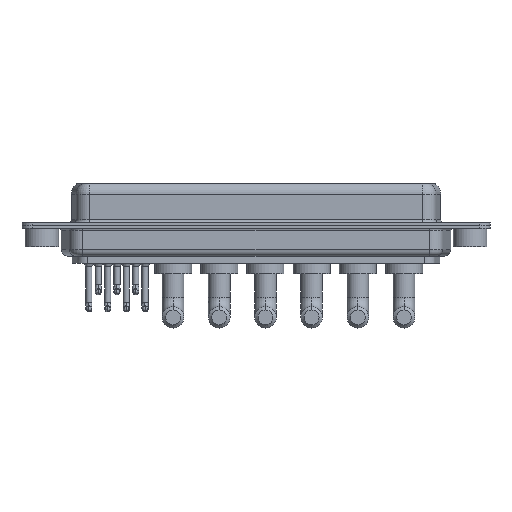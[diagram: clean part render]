
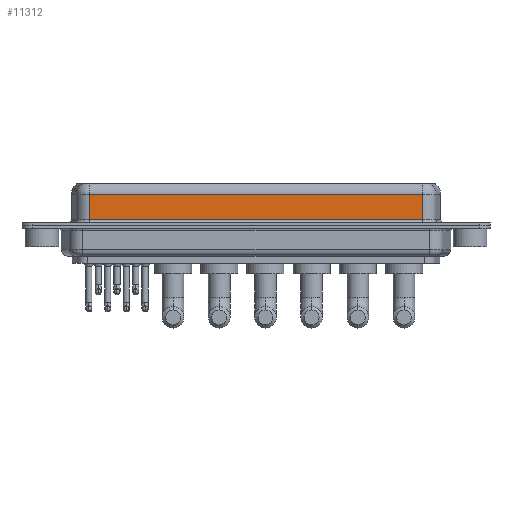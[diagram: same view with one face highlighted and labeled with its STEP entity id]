
A CAD part, front view. The second image highlights one B-rep face of the part: STEP entity #11312.
In plain terms, the highlighted planar face has unit normal (0, -1, 0).
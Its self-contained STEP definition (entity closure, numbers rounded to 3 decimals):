
#74 = LINE ( 'NONE', #2670, #17532 ) ;
#169 = VERTEX_POINT ( 'NONE', #14620 ) ;
#1276 = DIRECTION ( 'NONE',  ( 0., 0., -1. ) ) ;
#1426 = DIRECTION ( 'NONE',  ( -1., 0., 0. ) ) ;
#1740 = EDGE_CURVE ( 'NONE', #11932, #169, #18447, .T. ) ;
#2670 = CARTESIAN_POINT ( 'NONE',  ( 56.462, -3.95, 6.4 ) ) ;
#2834 = CARTESIAN_POINT ( 'NONE',  ( 56.462, -3.95, 4.65 ) ) ;
#3176 = VERTEX_POINT ( 'NONE', #13389 ) ;
#3404 = DIRECTION ( 'NONE',  ( 1., 0., 0. ) ) ;
#3586 = CARTESIAN_POINT ( 'NONE',  ( 56.462, -3.95, 0.9 ) ) ;
#4242 = VERTEX_POINT ( 'NONE', #7352 ) ;
#5449 = AXIS2_PLACEMENT_3D ( 'NONE', #15135, #15228, #6445 ) ;
#5517 = EDGE_CURVE ( 'NONE', #11932, #4242, #74, .T. ) ;
#5564 = EDGE_LOOP ( 'NONE', ( #15356, #7117, #18203, #12481 ) ) ;
#6445 = DIRECTION ( 'NONE',  ( 0., 0., 1. ) ) ;
#6584 = VECTOR ( 'NONE', #13882, 1000. ) ;
#7117 = ORIENTED_EDGE ( 'NONE', *, *, #1740, .T. ) ;
#7352 = CARTESIAN_POINT ( 'NONE',  ( 56.462, -3.95, 0.9 ) ) ;
#7949 = PLANE ( 'NONE',  #5449 ) ;
#8182 = EDGE_CURVE ( 'NONE', #169, #3176, #11280, .T. ) ;
#8204 = VECTOR ( 'NONE', #1426, 1000. ) ;
#8473 = EDGE_CURVE ( 'NONE', #3176, #4242, #16222, .T. ) ;
#9725 = FACE_OUTER_BOUND ( 'NONE', #5564, .T. ) ;
#11210 = CARTESIAN_POINT ( 'NONE',  ( 56.462, -3.95, 4.65 ) ) ;
#11280 = LINE ( 'NONE', #16697, #6584 ) ;
#11312 = ADVANCED_FACE ( 'NONE', ( #9725 ), #7949, .F. ) ;
#11932 = VERTEX_POINT ( 'NONE', #11210 ) ;
#12481 = ORIENTED_EDGE ( 'NONE', *, *, #8473, .T. ) ;
#13389 = CARTESIAN_POINT ( 'NONE',  ( 7.038, -3.95, 0.9 ) ) ;
#13882 = DIRECTION ( 'NONE',  ( 0., 0., -1. ) ) ;
#14327 = VECTOR ( 'NONE', #3404, 1000. ) ;
#14620 = CARTESIAN_POINT ( 'NONE',  ( 7.038, -3.95, 4.65 ) ) ;
#15135 = CARTESIAN_POINT ( 'NONE',  ( 56.462, -3.95, 6.4 ) ) ;
#15228 = DIRECTION ( 'NONE',  ( 0., 1., 0. ) ) ;
#15356 = ORIENTED_EDGE ( 'NONE', *, *, #5517, .F. ) ;
#16222 = LINE ( 'NONE', #3586, #14327 ) ;
#16697 = CARTESIAN_POINT ( 'NONE',  ( 7.038, -3.95, 6.4 ) ) ;
#17532 = VECTOR ( 'NONE', #1276, 1000. ) ;
#18203 = ORIENTED_EDGE ( 'NONE', *, *, #8182, .T. ) ;
#18447 = LINE ( 'NONE', #2834, #8204 ) ;
